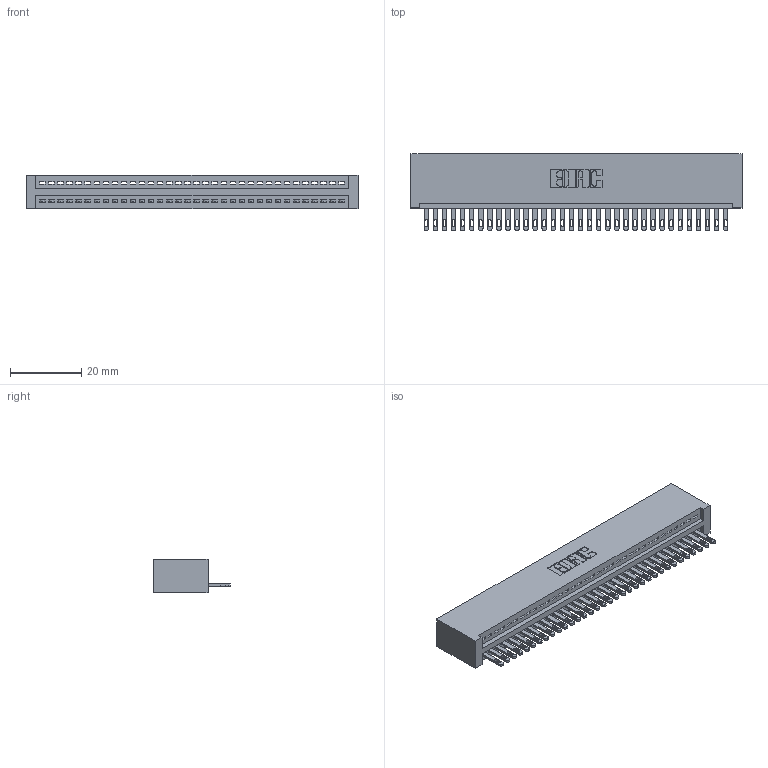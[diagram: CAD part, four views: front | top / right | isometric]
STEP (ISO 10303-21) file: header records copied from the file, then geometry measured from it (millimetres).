
FILE_DESCRIPTION (( 'STEP AP203' ), '1' );
FILE_NAME ('895-034-500-101.STEP', '2020-09-25T20:56:41', ( '' ), ( '' ), 'SwSTEP 2.0', 'SolidWorks 2020', '' );
FILE_SCHEMA (( 'CONFIG_CONTROL_DESIGN' ));
Length unit declared in the file: inch
Products named in the file (3): 345-292-001_345-293-100; 895-034-500-101; 845 Part_No Mounting Lugs
Assembly tree (35 placements, depth 2):
  895-034-500-101
    845 Part_No Mounting Lugs
    345-292-001_345-293-100  x34
Bounding box: 92.96 x 21.51 x 9.4 mm (x, y, z)
Volume: 9369.7 mm3; surface area: 12609.2 mm2
Topology: 35 solids, 35 shells, 1954 faces, 6029 edges, 4018 vertices
Faces by surface type: plane 1232, cylinder 722
Entity records: 26319 total; most frequent: CARTESIAN_POINT 4566, ORIENTED_EDGE 4534, DIRECTION 3995, EDGE_CURVE 2267, LINE 2003, VECTOR 2003, VERTEX_POINT 1510, AXIS2_PLACEMENT_3D 996
